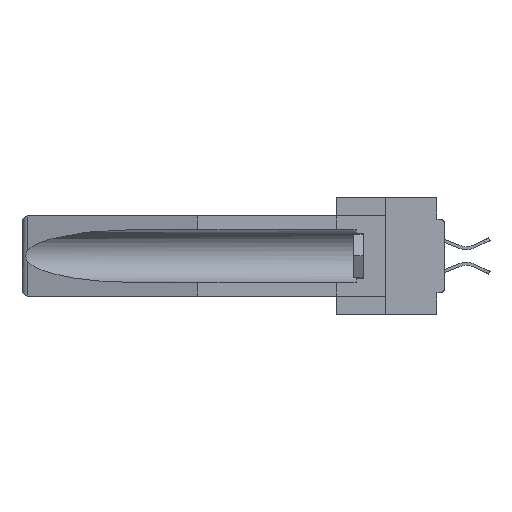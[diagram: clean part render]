
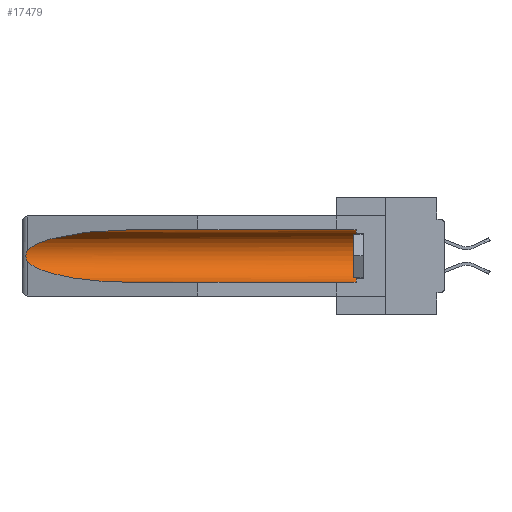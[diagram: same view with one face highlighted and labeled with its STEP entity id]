
A CAD part, left-side view. The second image highlights one B-rep face of the part: STEP entity #17479.
In plain terms, the highlighted cylindrical face has radius 2.857 mm (diameter 5.715 mm), a partial arc.
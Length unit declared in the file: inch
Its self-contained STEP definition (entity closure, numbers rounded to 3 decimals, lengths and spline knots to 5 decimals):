
#368 = EDGE_CURVE ( 'NONE', #3819, #27929, #18513, .T. ) ;
#1171 = CARTESIAN_POINT ( 'NONE',  ( 0.26537, 1.52718, -0.14972 ) ) ;
#1418 = FACE_OUTER_BOUND ( 'NONE', #29644, .T. ) ;
#1690 = EDGE_CURVE ( 'NONE', #22980, #20364, #19669, .T. ) ;
#2019 = DIRECTION ( 'NONE',  ( 0., 0., 1. ) ) ;
#2292 = CARTESIAN_POINT ( 'NONE',  ( 0.155, 0.126, -0.284 ) ) ;
#2359 = CYLINDRICAL_SURFACE ( 'NONE', #21159, 0.1125 ) ;
#2824 = CARTESIAN_POINT ( 'NONE',  ( 0.26537, 1.52718, -0.19328 ) ) ;
#3063 = ORIENTED_EDGE ( 'NONE', *, *, #368, .T. ) ;
#3255 = DIRECTION ( 'NONE',  ( 0., 0., 1. ) ) ;
#3819 = VERTEX_POINT ( 'NONE', #16416 ) ;
#3859 = CARTESIAN_POINT ( 'NONE',  ( 0.26537, 1.52718, -0.14972 ) ) ;
#4987 = B_SPLINE_CURVE_WITH_KNOTS ( 'NONE', 3,
 ( #35046, #20242, #15009, #20374, #20499, #26172, #29090, #29202, #5778, #2824 ),
 .UNSPECIFIED., .F., .F.,
 ( 4, 2, 2, 2, 4 ),
 ( 0., 0.00029, 0.00058, 0.00087, 0.00117 ),
 .UNSPECIFIED. ) ;
#5778 = CARTESIAN_POINT ( 'NONE',  ( 0.26597, 1.5296, -0.19026 ) ) ;
#7161 = EDGE_CURVE ( 'NONE', #27929, #22980, #4987, .T. ) ;
#7540 = VERTEX_POINT ( 'NONE', #2292 ) ;
#8209 = CARTESIAN_POINT ( 'NONE',  ( 0.26537, 1.52718, -0.19328 ) ) ;
#9112 = CARTESIAN_POINT ( 'NONE',  ( 0.25451, 1.48313, -0.24835 ) ) ;
#10809 = CARTESIAN_POINT ( 'NONE',  ( 0.155, 0.126, -0.1715 ) ) ;
#11004 = VERTEX_POINT ( 'NONE', #21621 ) ;
#11611 = DIRECTION ( 'NONE',  ( 0., 1., 0. ) ) ;
#11679 = CARTESIAN_POINT ( 'NONE',  ( 0.155, 1.07973, -0.284 ) ) ;
#11680 = DIRECTION ( 'NONE',  ( 0., 1., 0. ) ) ;
#13625 = LINE ( 'NONE', #37052, #15031 ) ;
#15009 = CARTESIAN_POINT ( 'NONE',  ( 0.26654, 1.53092, -0.15636 ) ) ;
#15031 = VECTOR ( 'NONE', #11611, 39.37008 ) ;
#15671 = CARTESIAN_POINT ( 'NONE',  ( 0.155, 1.07973, -0.059 ) ) ;
#16416 = CARTESIAN_POINT ( 'NONE',  ( 0.155, 1.07973, -0.059 ) ) ;
#17479 = ADVANCED_FACE ( 'NONE', ( #1418 ), #2359, .F. ) ;
#18513 =( BOUNDED_CURVE ( )  B_SPLINE_CURVE ( 3, ( #15671, #21369, #27461, #1171 ),
 .UNSPECIFIED., .F., .F. ) 
 B_SPLINE_CURVE_WITH_KNOTS ( ( 4, 4 ),
 ( 4.71239, 6.08839 ),
 .UNSPECIFIED. ) 
 CURVE ( )  GEOMETRIC_REPRESENTATION_ITEM ( )  RATIONAL_B_SPLINE_CURVE ( ( 1., 0.848, 0.848, 1. ) ) 
 REPRESENTATION_ITEM ( '' )  );
#18811 = CARTESIAN_POINT ( 'NONE',  ( 0.155, -0.30754, -0.284 ) ) ;
#19422 = EDGE_CURVE ( 'NONE', #7540, #20364, #36270, .T. ) ;
#19669 =( BOUNDED_CURVE ( )  B_SPLINE_CURVE ( 3, ( #31950, #9112, #32203, #11679 ),
 .UNSPECIFIED., .F., .F. ) 
 B_SPLINE_CURVE_WITH_KNOTS ( ( 4, 4 ),
 ( 0.1948, 1.5708 ),
 .UNSPECIFIED. ) 
 CURVE ( )  GEOMETRIC_REPRESENTATION_ITEM ( )  RATIONAL_B_SPLINE_CURVE ( ( 1., 0.848, 0.848, 1. ) ) 
 REPRESENTATION_ITEM ( '' )  );
#20060 = CIRCLE ( 'NONE', #27386, 0.1125 ) ;
#20242 = CARTESIAN_POINT ( 'NONE',  ( 0.26597, 1.52961, -0.15275 ) ) ;
#20364 = VERTEX_POINT ( 'NONE', #35983 ) ;
#20374 = CARTESIAN_POINT ( 'NONE',  ( 0.2673, 1.5327, -0.16383 ) ) ;
#20499 = CARTESIAN_POINT ( 'NONE',  ( 0.2675, 1.53308, -0.16763 ) ) ;
#21159 = AXIS2_PLACEMENT_3D ( 'NONE', #26128, #11680, #3255 ) ;
#21369 = CARTESIAN_POINT ( 'NONE',  ( 0.21114, 1.30732, -0.059 ) ) ;
#21432 = DIRECTION ( 'NONE',  ( 0., 1., 0. ) ) ;
#21621 = CARTESIAN_POINT ( 'NONE',  ( 0.155, 0.126, -0.059 ) ) ;
#22830 = DIRECTION ( 'NONE',  ( 0., -1., 0. ) ) ;
#22980 = VERTEX_POINT ( 'NONE', #8209 ) ;
#24197 = ORIENTED_EDGE ( 'NONE', *, *, #19422, .F. ) ;
#26128 = CARTESIAN_POINT ( 'NONE',  ( 0.155, -0.30754, -0.1715 ) ) ;
#26172 = CARTESIAN_POINT ( 'NONE',  ( 0.2675, 1.53308, -0.17534 ) ) ;
#27386 = AXIS2_PLACEMENT_3D ( 'NONE', #10809, #22830, #2019 ) ;
#27461 = CARTESIAN_POINT ( 'NONE',  ( 0.25451, 1.48313, -0.09465 ) ) ;
#27834 = ORIENTED_EDGE ( 'NONE', *, *, #33662, .T. ) ;
#27929 = VERTEX_POINT ( 'NONE', #3859 ) ;
#28384 = EDGE_CURVE ( 'NONE', #11004, #3819, #13625, .T. ) ;
#28597 = ORIENTED_EDGE ( 'NONE', *, *, #1690, .T. ) ;
#29090 = CARTESIAN_POINT ( 'NONE',  ( 0.2673, 1.53269, -0.17917 ) ) ;
#29202 = CARTESIAN_POINT ( 'NONE',  ( 0.26655, 1.53094, -0.18657 ) ) ;
#29644 = EDGE_LOOP ( 'NONE', ( #3063, #36719, #28597, #24197, #27834, #37019 ) ) ;
#30395 = VECTOR ( 'NONE', #21432, 39.37008 ) ;
#31950 = CARTESIAN_POINT ( 'NONE',  ( 0.26537, 1.52718, -0.19328 ) ) ;
#32203 = CARTESIAN_POINT ( 'NONE',  ( 0.21114, 1.30732, -0.284 ) ) ;
#33662 = EDGE_CURVE ( 'NONE', #7540, #11004, #20060, .T. ) ;
#35046 = CARTESIAN_POINT ( 'NONE',  ( 0.26537, 1.52718, -0.14972 ) ) ;
#35983 = CARTESIAN_POINT ( 'NONE',  ( 0.155, 1.07973, -0.284 ) ) ;
#36270 = LINE ( 'NONE', #18811, #30395 ) ;
#36719 = ORIENTED_EDGE ( 'NONE', *, *, #7161, .T. ) ;
#37019 = ORIENTED_EDGE ( 'NONE', *, *, #28384, .T. ) ;
#37052 = CARTESIAN_POINT ( 'NONE',  ( 0.155, -0.30754, -0.059 ) ) ;
